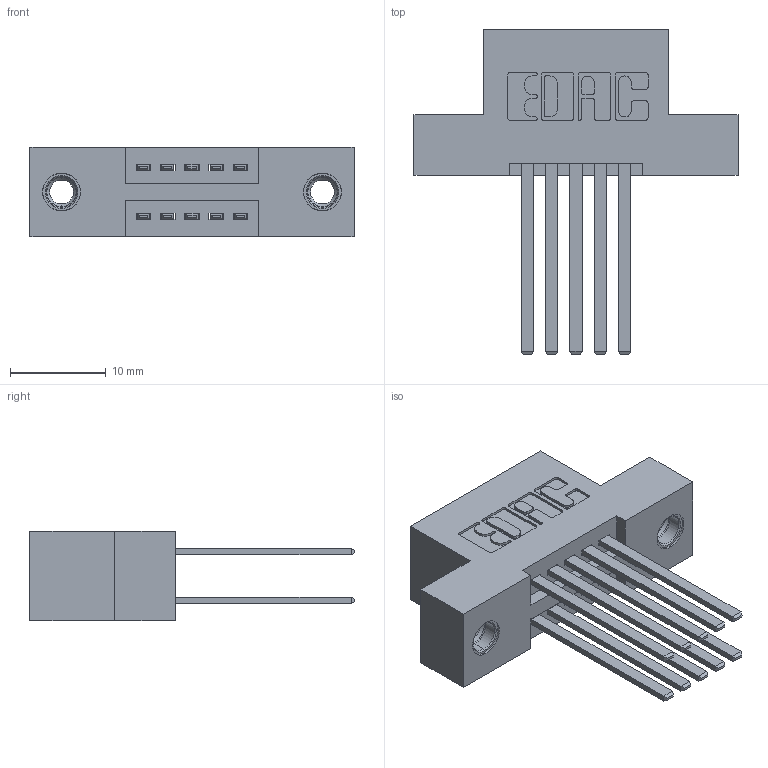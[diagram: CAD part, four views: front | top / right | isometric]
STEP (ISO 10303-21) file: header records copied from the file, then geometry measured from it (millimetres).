
FILE_DESCRIPTION (( 'STEP AP203' ), '1' );
FILE_NAME ('395-010-544-207.STEP', '2019-10-15T11:49:11', ( '' ), ( '' ), 'SwSTEP 2.0', 'SolidWorks 2016', '' );
FILE_SCHEMA (( 'CONFIG_CONTROL_DESIGN' ));
Length unit declared in the file: inch
Products named in the file (4): 345-250-001_345-250-005-103; 395-010-544-207; 345 Part_Flush Mounting Lugs - 0.156 Dia-TI; 345-292-001_345-293-144
Assembly tree (13 placements, depth 2):
  395-010-544-207
    345 Part_Flush Mounting Lugs - 0.156 Dia-TI
    345-292-001_345-293-144  x10
    345-250-001_345-250-005-103  x2
Bounding box: 33.91 x 33.96 x 9.4 mm (x, y, z)
Volume: 3077.2 mm3; surface area: 4270.7 mm2
Topology: 13 solids, 13 shells, 626 faces, 1787 edges, 1170 vertices
Faces by surface type: plane 402, cylinder 208, cone 12, torus 4
Entity records: 9906 total; most frequent: CARTESIAN_POINT 1675, ORIENTED_EDGE 1602, DIRECTION 1547, EDGE_CURVE 801, LINE 633, VECTOR 633, VERTEX_POINT 528, AXIS2_PLACEMENT_3D 457
